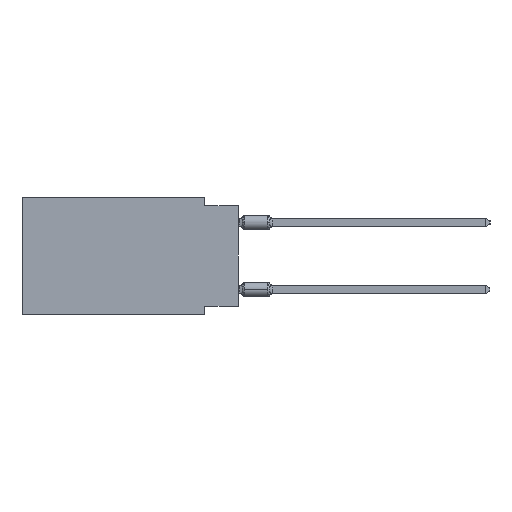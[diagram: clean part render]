
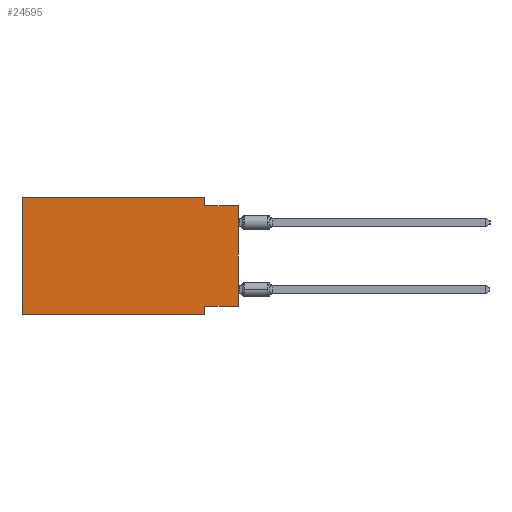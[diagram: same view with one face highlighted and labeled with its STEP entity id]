
A CAD part, left-side view. The second image highlights one B-rep face of the part: STEP entity #24595.
In plain terms, the highlighted planar face has unit normal (-1, 0, 0).
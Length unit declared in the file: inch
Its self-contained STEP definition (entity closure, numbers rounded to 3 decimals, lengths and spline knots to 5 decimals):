
#1125 = VERTEX_POINT ( 'NONE', #41177 ) ;
#1634 = VECTOR ( 'NONE', #11792, 39.37008 ) ;
#4071 = CARTESIAN_POINT ( 'NONE',  ( 0., 0.645, -0.35 ) ) ;
#4763 = VECTOR ( 'NONE', #20294, 39.37008 ) ;
#5988 = CARTESIAN_POINT ( 'NONE',  ( 0., 0.1, 0. ) ) ;
#7477 = CARTESIAN_POINT ( 'NONE',  ( 0., 0., -0.025 ) ) ;
#9595 = ORIENTED_EDGE ( 'NONE', *, *, #38094, .F. ) ;
#10442 = EDGE_CURVE ( 'NONE', #1125, #54634, #47152, .T. ) ;
#10838 = LINE ( 'NONE', #5988, #4763 ) ;
#11792 = DIRECTION ( 'NONE',  ( 0., -1., 0. ) ) ;
#14010 = CARTESIAN_POINT ( 'NONE',  ( 0., 0., -0.025 ) ) ;
#14482 = CARTESIAN_POINT ( 'NONE',  ( 0., 0.645, 0. ) ) ;
#15599 = EDGE_CURVE ( 'NONE', #54336, #1125, #16538, .T. ) ;
#16475 = VERTEX_POINT ( 'NONE', #45020 ) ;
#16538 = LINE ( 'NONE', #50341, #26334 ) ;
#16578 = VECTOR ( 'NONE', #52023, 39.37008 ) ;
#17965 = CARTESIAN_POINT ( 'NONE',  ( 0., 0.645, 0. ) ) ;
#18452 = ORIENTED_EDGE ( 'NONE', *, *, #58636, .F. ) ;
#18889 = CARTESIAN_POINT ( 'NONE',  ( 0., 0., 0. ) ) ;
#19273 = PLANE ( 'NONE',  #59254 ) ;
#20294 = DIRECTION ( 'NONE',  ( 0., 0., -1. ) ) ;
#24577 = VECTOR ( 'NONE', #57640, 39.37008 ) ;
#24595 = ADVANCED_FACE ( 'NONE', ( #48801 ), #19273, .F. ) ;
#26334 = VECTOR ( 'NONE', #45169, 39.37008 ) ;
#28548 = ORIENTED_EDGE ( 'NONE', *, *, #58510, .F. ) ;
#28804 = CARTESIAN_POINT ( 'NONE',  ( 0., 0., -0.325 ) ) ;
#31356 = VECTOR ( 'NONE', #33849, 39.37008 ) ;
#31501 = EDGE_CURVE ( 'NONE', #34922, #54339, #56682, .T. ) ;
#32340 = CARTESIAN_POINT ( 'NONE',  ( 0., 0.645, 0. ) ) ;
#33469 = ORIENTED_EDGE ( 'NONE', *, *, #31501, .F. ) ;
#33846 = LINE ( 'NONE', #18889, #56123 ) ;
#33849 = DIRECTION ( 'NONE',  ( 0., -1., 0. ) ) ;
#34491 = LINE ( 'NONE', #14010, #31356 ) ;
#34922 = VERTEX_POINT ( 'NONE', #4071 ) ;
#37328 = ORIENTED_EDGE ( 'NONE', *, *, #51861, .T. ) ;
#38094 = EDGE_CURVE ( 'NONE', #40553, #61519, #34491, .T. ) ;
#39085 = DIRECTION ( 'NONE',  ( 1., 0., 0. ) ) ;
#40553 = VERTEX_POINT ( 'NONE', #50755 ) ;
#41068 = DIRECTION ( 'NONE',  ( 0., -1., 0. ) ) ;
#41177 = CARTESIAN_POINT ( 'NONE',  ( 0., 0.1, -0.325 ) ) ;
#42291 = CARTESIAN_POINT ( 'NONE',  ( 0., 0.1, -0.35 ) ) ;
#42354 = CARTESIAN_POINT ( 'NONE',  ( 0., 0.1, -0.35 ) ) ;
#42905 = EDGE_LOOP ( 'NONE', ( #37328, #9595, #28548, #18452, #33469, #62086, #53555, #52132 ) ) ;
#43252 = DIRECTION ( 'NONE',  ( 0., 0., 1. ) ) ;
#43300 = DIRECTION ( 'NONE',  ( 0., 0., -1. ) ) ;
#45020 = CARTESIAN_POINT ( 'NONE',  ( 0., 0.1, 0. ) ) ;
#45169 = DIRECTION ( 'NONE',  ( 0., 1., 0. ) ) ;
#45284 = VECTOR ( 'NONE', #41068, 39.37008 ) ;
#47152 = LINE ( 'NONE', #42291, #16578 ) ;
#48801 = FACE_OUTER_BOUND ( 'NONE', #42905, .T. ) ;
#50341 = CARTESIAN_POINT ( 'NONE',  ( 0., 0., -0.325 ) ) ;
#50755 = CARTESIAN_POINT ( 'NONE',  ( 0., 0.1, -0.025 ) ) ;
#50789 = LINE ( 'NONE', #55033, #45284 ) ;
#51861 = EDGE_CURVE ( 'NONE', #54336, #61519, #33846, .T. ) ;
#52023 = DIRECTION ( 'NONE',  ( 0., 0., -1. ) ) ;
#52132 = ORIENTED_EDGE ( 'NONE', *, *, #15599, .F. ) ;
#52690 = CARTESIAN_POINT ( 'NONE',  ( 0., 0.645, 0. ) ) ;
#53555 = ORIENTED_EDGE ( 'NONE', *, *, #10442, .F. ) ;
#54336 = VERTEX_POINT ( 'NONE', #28804 ) ;
#54339 = VERTEX_POINT ( 'NONE', #14482 ) ;
#54634 = VERTEX_POINT ( 'NONE', #42354 ) ;
#55033 = CARTESIAN_POINT ( 'NONE',  ( 0., 0.645, -0.35 ) ) ;
#56123 = VECTOR ( 'NONE', #43252, 39.37008 ) ;
#56682 = LINE ( 'NONE', #32340, #24577 ) ;
#56927 = LINE ( 'NONE', #52690, #1634 ) ;
#57640 = DIRECTION ( 'NONE',  ( 0., 0., 1. ) ) ;
#58510 = EDGE_CURVE ( 'NONE', #16475, #40553, #10838, .T. ) ;
#58636 = EDGE_CURVE ( 'NONE', #54339, #16475, #56927, .T. ) ;
#59254 = AXIS2_PLACEMENT_3D ( 'NONE', #17965, #39085, #43300 ) ;
#59792 = EDGE_CURVE ( 'NONE', #34922, #54634, #50789, .T. ) ;
#61519 = VERTEX_POINT ( 'NONE', #7477 ) ;
#62086 = ORIENTED_EDGE ( 'NONE', *, *, #59792, .T. ) ;
